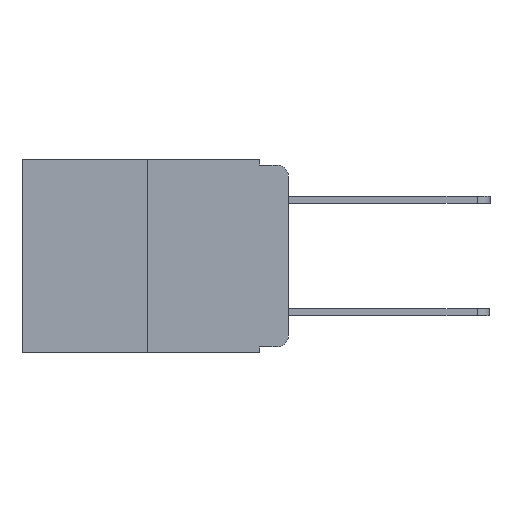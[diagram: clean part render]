
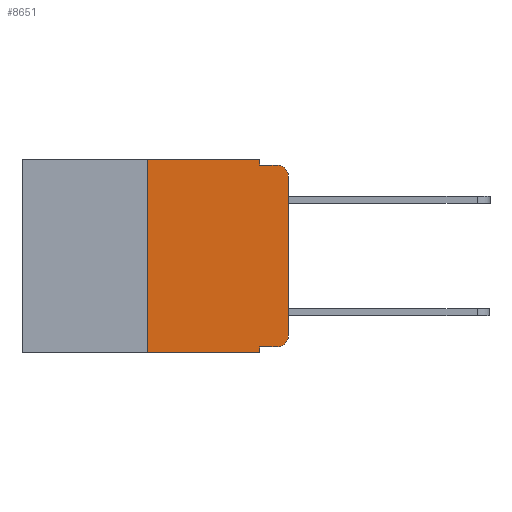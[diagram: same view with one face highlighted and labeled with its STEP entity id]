
A CAD part, left-side view. The second image highlights one B-rep face of the part: STEP entity #8651.
In plain terms, the highlighted planar face has unit normal (-1, 0, 0).
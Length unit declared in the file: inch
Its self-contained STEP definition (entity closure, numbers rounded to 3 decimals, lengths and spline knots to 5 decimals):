
#173 = VERTEX_POINT ( 'NONE', #7905 ) ;
#272 = AXIS2_PLACEMENT_3D ( 'NONE', #2808, #5011, #4977 ) ;
#518 = DIRECTION ( 'NONE',  ( 0., 0., -1. ) ) ;
#750 = CARTESIAN_POINT ( 'NONE',  ( 0., 0.051, -0.343 ) ) ;
#1056 = EDGE_CURVE ( 'NONE', #8119, #173, #10871, .T. ) ;
#1078 = CARTESIAN_POINT ( 'NONE',  ( 0., 0., 0. ) ) ;
#1331 = CIRCLE ( 'NONE', #272, 0.02 ) ;
#1340 = VECTOR ( 'NONE', #9763, 39.37008 ) ;
#1777 = EDGE_LOOP ( 'NONE', ( #6140, #8580, #2374, #8888, #11629, #11385, #2017, #2556, #7523, #5688 ) ) ;
#1946 = DIRECTION ( 'NONE',  ( 0., -1., 0. ) ) ;
#2017 = ORIENTED_EDGE ( 'NONE', *, *, #3315, .T. ) ;
#2068 = EDGE_CURVE ( 'NONE', #5308, #6868, #10874, .T. ) ;
#2088 = EDGE_CURVE ( 'NONE', #173, #6345, #6199, .T. ) ;
#2121 = EDGE_CURVE ( 'NONE', #6345, #9777, #7649, .T. ) ;
#2253 = EDGE_CURVE ( 'NONE', #3209, #5308, #10634, .T. ) ;
#2260 = EDGE_CURVE ( 'NONE', #6868, #9777, #1331, .T. ) ;
#2326 = EDGE_CURVE ( 'NONE', #2912, #3209, #11631, .T. ) ;
#2372 = VECTOR ( 'NONE', #2795, 39.37008 ) ;
#2374 = ORIENTED_EDGE ( 'NONE', *, *, #2121, .F. ) ;
#2378 = EDGE_CURVE ( 'NONE', #2912, #9054, #4240, .T. ) ;
#2404 = EDGE_CURVE ( 'NONE', #2961, #8119, #8033, .T. ) ;
#2479 = CARTESIAN_POINT ( 'NONE',  ( 0., 0.473, 0. ) ) ;
#2510 = CARTESIAN_POINT ( 'NONE',  ( 0., 0.051, 0. ) ) ;
#2556 = ORIENTED_EDGE ( 'NONE', *, *, #2378, .F. ) ;
#2795 = DIRECTION ( 'NONE',  ( 0., -1., 0. ) ) ;
#2808 = CARTESIAN_POINT ( 'NONE',  ( 0., 0.02, -0.03 ) ) ;
#2912 = VERTEX_POINT ( 'NONE', #5180 ) ;
#2961 = VERTEX_POINT ( 'NONE', #4033 ) ;
#3105 = CARTESIAN_POINT ( 'NONE',  ( 0., 0.02, -0.333 ) ) ;
#3209 = VERTEX_POINT ( 'NONE', #3105 ) ;
#3315 = EDGE_CURVE ( 'NONE', #2961, #9054, #9508, .T. ) ;
#4033 = CARTESIAN_POINT ( 'NONE',  ( 0., 0.25, -0.343 ) ) ;
#4127 = VECTOR ( 'NONE', #9893, 39.37008 ) ;
#4240 = LINE ( 'NONE', #2510, #6310 ) ;
#4417 = PLANE ( 'NONE',  #7128 ) ;
#4929 = CARTESIAN_POINT ( 'NONE',  ( 0., 0.051, -0.333 ) ) ;
#4977 = DIRECTION ( 'NONE',  ( 0., 0., -1. ) ) ;
#5011 = DIRECTION ( 'NONE',  ( -1., 0., 0. ) ) ;
#5047 = CARTESIAN_POINT ( 'NONE',  ( 0., 0.25, 0. ) ) ;
#5180 = CARTESIAN_POINT ( 'NONE',  ( 0., 0.051, -0.333 ) ) ;
#5272 = CARTESIAN_POINT ( 'NONE',  ( 0., 0.02, -0.313 ) ) ;
#5300 = DIRECTION ( 'NONE',  ( 1., 0., 0. ) ) ;
#5308 = VERTEX_POINT ( 'NONE', #10757 ) ;
#5328 = DIRECTION ( 'NONE',  ( 0., 0., -1. ) ) ;
#5400 = DIRECTION ( 'NONE',  ( -1., 0., 0. ) ) ;
#5688 = ORIENTED_EDGE ( 'NONE', *, *, #2253, .T. ) ;
#5914 = VECTOR ( 'NONE', #7651, 39.37008 ) ;
#5939 = DIRECTION ( 'NONE',  ( 0., -1., 0. ) ) ;
#6140 = ORIENTED_EDGE ( 'NONE', *, *, #2068, .T. ) ;
#6199 = LINE ( 'NONE', #7687, #5914 ) ;
#6310 = VECTOR ( 'NONE', #518, 39.37008 ) ;
#6345 = VERTEX_POINT ( 'NONE', #10644 ) ;
#6750 = CARTESIAN_POINT ( 'NONE',  ( 0., 0.051, -0.01 ) ) ;
#6868 = VERTEX_POINT ( 'NONE', #7896 ) ;
#7087 = VECTOR ( 'NONE', #1946, 39.37008 ) ;
#7128 = AXIS2_PLACEMENT_3D ( 'NONE', #2479, #5300, #11133 ) ;
#7523 = ORIENTED_EDGE ( 'NONE', *, *, #2326, .T. ) ;
#7574 = CARTESIAN_POINT ( 'NONE',  ( 0., 0.473, -0.343 ) ) ;
#7649 = LINE ( 'NONE', #6750, #11434 ) ;
#7651 = DIRECTION ( 'NONE',  ( 0., 0., -1. ) ) ;
#7687 = CARTESIAN_POINT ( 'NONE',  ( 0., 0.051, 0. ) ) ;
#7761 = CARTESIAN_POINT ( 'NONE',  ( 0., 0.473, 0. ) ) ;
#7770 = VECTOR ( 'NONE', #11108, 39.37008 ) ;
#7809 = CARTESIAN_POINT ( 'NONE',  ( 0., 0.25, 0. ) ) ;
#7896 = CARTESIAN_POINT ( 'NONE',  ( 0., 0., -0.03 ) ) ;
#7905 = CARTESIAN_POINT ( 'NONE',  ( 0., 0.051, 0. ) ) ;
#8033 = LINE ( 'NONE', #7809, #7770 ) ;
#8119 = VERTEX_POINT ( 'NONE', #5047 ) ;
#8580 = ORIENTED_EDGE ( 'NONE', *, *, #2260, .T. ) ;
#8651 = ADVANCED_FACE ( 'NONE', ( #10931 ), #4417, .F. ) ;
#8888 = ORIENTED_EDGE ( 'NONE', *, *, #2088, .F. ) ;
#9054 = VERTEX_POINT ( 'NONE', #750 ) ;
#9508 = LINE ( 'NONE', #7574, #2372 ) ;
#9763 = DIRECTION ( 'NONE',  ( 0., 0., 1. ) ) ;
#9777 = VERTEX_POINT ( 'NONE', #10092 ) ;
#9893 = DIRECTION ( 'NONE',  ( 0., -1., 0. ) ) ;
#10092 = CARTESIAN_POINT ( 'NONE',  ( 0., 0.02, -0.01 ) ) ;
#10634 = CIRCLE ( 'NONE', #11442, 0.02 ) ;
#10644 = CARTESIAN_POINT ( 'NONE',  ( 0., 0.051, -0.01 ) ) ;
#10757 = CARTESIAN_POINT ( 'NONE',  ( 0., 0., -0.313 ) ) ;
#10871 = LINE ( 'NONE', #7761, #4127 ) ;
#10874 = LINE ( 'NONE', #1078, #1340 ) ;
#10931 = FACE_OUTER_BOUND ( 'NONE', #1777, .T. ) ;
#11108 = DIRECTION ( 'NONE',  ( 0., 0., 1. ) ) ;
#11133 = DIRECTION ( 'NONE',  ( 0., 0., -1. ) ) ;
#11385 = ORIENTED_EDGE ( 'NONE', *, *, #2404, .F. ) ;
#11434 = VECTOR ( 'NONE', #5939, 39.37008 ) ;
#11442 = AXIS2_PLACEMENT_3D ( 'NONE', #5272, #5400, #5328 ) ;
#11629 = ORIENTED_EDGE ( 'NONE', *, *, #1056, .F. ) ;
#11631 = LINE ( 'NONE', #4929, #7087 ) ;
